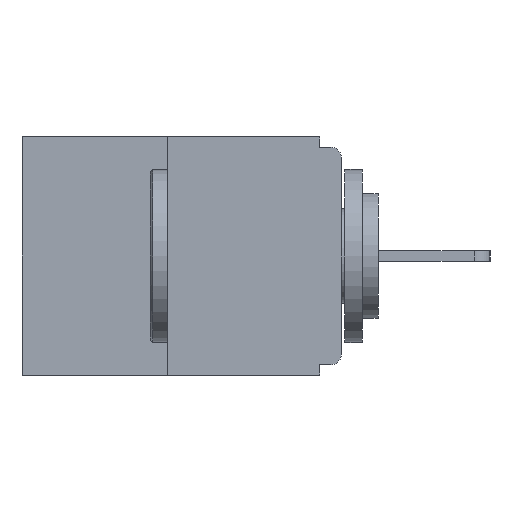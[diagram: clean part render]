
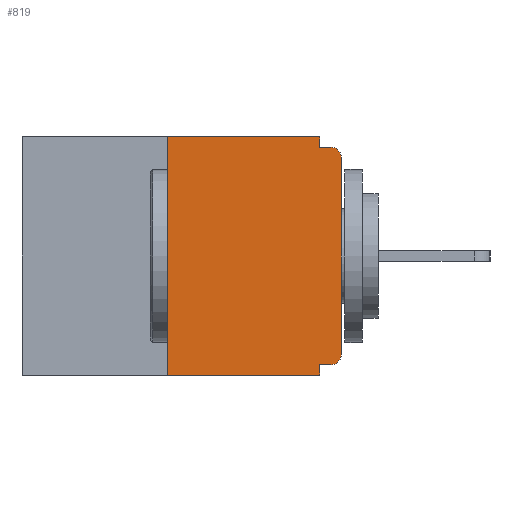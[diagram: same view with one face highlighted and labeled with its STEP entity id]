
A CAD part, left-side view. The second image highlights one B-rep face of the part: STEP entity #819.
In plain terms, the highlighted planar face has unit normal (-1, 0, 0).
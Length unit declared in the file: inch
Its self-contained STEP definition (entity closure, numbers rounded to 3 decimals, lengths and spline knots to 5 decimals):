
#14 = ORIENTED_EDGE ( 'NONE', *, *, #9934, .F. ) ;
#819 = ADVANCED_FACE ( 'NONE', ( #9322 ), #13256, .F. ) ;
#876 = ORIENTED_EDGE ( 'NONE', *, *, #11588, .F. ) ;
#1286 = LINE ( 'NONE', #10309, #9996 ) ;
#1894 = CARTESIAN_POINT ( 'NONE',  ( 0., 0., -0.015 ) ) ;
#1995 = DIRECTION ( 'NONE',  ( 0., 1., 0. ) ) ;
#2075 = EDGE_CURVE ( 'NONE', #4743, #5953, #8458, .T. ) ;
#2140 = ORIENTED_EDGE ( 'NONE', *, *, #2527, .F. ) ;
#2394 = CARTESIAN_POINT ( 'NONE',  ( 0., 0.015, -0.313 ) ) ;
#2504 = VERTEX_POINT ( 'NONE', #10908 ) ;
#2527 = EDGE_CURVE ( 'NONE', #2734, #2504, #3338, .T. ) ;
#2647 = CIRCLE ( 'NONE', #12178, 0.015 ) ;
#2734 = VERTEX_POINT ( 'NONE', #10225 ) ;
#2845 = DIRECTION ( 'NONE',  ( 0., 0., -1. ) ) ;
#3244 = ORIENTED_EDGE ( 'NONE', *, *, #14986, .T. ) ;
#3322 = EDGE_CURVE ( 'NONE', #6331, #4894, #5520, .T. ) ;
#3338 = LINE ( 'NONE', #15230, #3582 ) ;
#3570 = CARTESIAN_POINT ( 'NONE',  ( 0., 0.015, -0.015 ) ) ;
#3582 = VECTOR ( 'NONE', #4442, 39.37008 ) ;
#3686 = DIRECTION ( 'NONE',  ( 0., -1., 0. ) ) ;
#3783 = EDGE_CURVE ( 'NONE', #7012, #4894, #4788, .T. ) ;
#4094 = VECTOR ( 'NONE', #6045, 39.37008 ) ;
#4170 = CARTESIAN_POINT ( 'NONE',  ( 0., 0.031, -0.328 ) ) ;
#4374 = CARTESIAN_POINT ( 'NONE',  ( 0., 0.46, -0.343 ) ) ;
#4442 = DIRECTION ( 'NONE',  ( 0., 0., 1. ) ) ;
#4688 = ORIENTED_EDGE ( 'NONE', *, *, #3783, .F. ) ;
#4743 = VERTEX_POINT ( 'NONE', #10892 ) ;
#4788 = LINE ( 'NONE', #1894, #4094 ) ;
#4894 = VERTEX_POINT ( 'NONE', #3570 ) ;
#5467 = DIRECTION ( 'NONE',  ( 1., 0., 0. ) ) ;
#5520 = CIRCLE ( 'NONE', #15119, 0.015 ) ;
#5645 = DIRECTION ( 'NONE',  ( 0., -1., 0. ) ) ;
#5673 = VERTEX_POINT ( 'NONE', #12228 ) ;
#5953 = VERTEX_POINT ( 'NONE', #4170 ) ;
#6045 = DIRECTION ( 'NONE',  ( 0., -1., 0. ) ) ;
#6171 = VERTEX_POINT ( 'NONE', #7486 ) ;
#6331 = VERTEX_POINT ( 'NONE', #14590 ) ;
#6873 = CARTESIAN_POINT ( 'NONE',  ( 0., 0.031, 0. ) ) ;
#6968 = LINE ( 'NONE', #6873, #16480 ) ;
#7012 = VERTEX_POINT ( 'NONE', #16788 ) ;
#7073 = CARTESIAN_POINT ( 'NONE',  ( 0., 0.031, 0. ) ) ;
#7255 = VECTOR ( 'NONE', #5645, 39.37008 ) ;
#7283 = ORIENTED_EDGE ( 'NONE', *, *, #3322, .T. ) ;
#7486 = CARTESIAN_POINT ( 'NONE',  ( 0., 0.031, -0.343 ) ) ;
#7665 = AXIS2_PLACEMENT_3D ( 'NONE', #14556, #5467, #2845 ) ;
#7967 = CARTESIAN_POINT ( 'NONE',  ( 0., 0.015, -0.03 ) ) ;
#8371 = LINE ( 'NONE', #13602, #9650 ) ;
#8458 = LINE ( 'NONE', #11026, #11518 ) ;
#8956 = ORIENTED_EDGE ( 'NONE', *, *, #14340, .T. ) ;
#8972 = EDGE_CURVE ( 'NONE', #14703, #7012, #6968, .T. ) ;
#9206 = DIRECTION ( 'NONE',  ( 0., 0., -1. ) ) ;
#9322 = FACE_OUTER_BOUND ( 'NONE', #11728, .T. ) ;
#9346 = DIRECTION ( 'NONE',  ( -1., 0., 0. ) ) ;
#9544 = DIRECTION ( 'NONE',  ( 0., 0., -1. ) ) ;
#9650 = VECTOR ( 'NONE', #9747, 39.37008 ) ;
#9747 = DIRECTION ( 'NONE',  ( 0., 0., -1. ) ) ;
#9934 = EDGE_CURVE ( 'NONE', #2504, #14703, #11424, .T. ) ;
#9996 = VECTOR ( 'NONE', #15647, 39.37008 ) ;
#10201 = VECTOR ( 'NONE', #3686, 39.37008 ) ;
#10225 = CARTESIAN_POINT ( 'NONE',  ( 0., 0.25, -0.343 ) ) ;
#10309 = CARTESIAN_POINT ( 'NONE',  ( 0., 0., 0. ) ) ;
#10364 = DIRECTION ( 'NONE',  ( 0., 0., -1. ) ) ;
#10892 = CARTESIAN_POINT ( 'NONE',  ( 0., 0.015, -0.328 ) ) ;
#10908 = CARTESIAN_POINT ( 'NONE',  ( 0., 0.25, 0. ) ) ;
#11026 = CARTESIAN_POINT ( 'NONE',  ( 0., 0., -0.328 ) ) ;
#11424 = LINE ( 'NONE', #15649, #10201 ) ;
#11518 = VECTOR ( 'NONE', #1995, 39.37008 ) ;
#11588 = EDGE_CURVE ( 'NONE', #5953, #6171, #8371, .T. ) ;
#11728 = EDGE_LOOP ( 'NONE', ( #14, #2140, #8956, #876, #16757, #3244, #13403, #7283, #4688, #14796 ) ) ;
#11966 = LINE ( 'NONE', #4374, #7255 ) ;
#12178 = AXIS2_PLACEMENT_3D ( 'NONE', #2394, #13330, #9206 ) ;
#12228 = CARTESIAN_POINT ( 'NONE',  ( 0., 0., -0.313 ) ) ;
#13256 = PLANE ( 'NONE',  #7665 ) ;
#13330 = DIRECTION ( 'NONE',  ( -1., 0., 0. ) ) ;
#13403 = ORIENTED_EDGE ( 'NONE', *, *, #16213, .T. ) ;
#13602 = CARTESIAN_POINT ( 'NONE',  ( 0., 0.031, -0.343 ) ) ;
#14340 = EDGE_CURVE ( 'NONE', #2734, #6171, #11966, .T. ) ;
#14556 = CARTESIAN_POINT ( 'NONE',  ( 0., 0.46, 0. ) ) ;
#14590 = CARTESIAN_POINT ( 'NONE',  ( 0., 0., -0.03 ) ) ;
#14703 = VERTEX_POINT ( 'NONE', #7073 ) ;
#14796 = ORIENTED_EDGE ( 'NONE', *, *, #8972, .F. ) ;
#14986 = EDGE_CURVE ( 'NONE', #4743, #5673, #2647, .T. ) ;
#15119 = AXIS2_PLACEMENT_3D ( 'NONE', #7967, #9346, #10364 ) ;
#15230 = CARTESIAN_POINT ( 'NONE',  ( 0., 0.25, 0. ) ) ;
#15647 = DIRECTION ( 'NONE',  ( 0., 0., 1. ) ) ;
#15649 = CARTESIAN_POINT ( 'NONE',  ( 0., 0.46, 0. ) ) ;
#16213 = EDGE_CURVE ( 'NONE', #5673, #6331, #1286, .T. ) ;
#16480 = VECTOR ( 'NONE', #9544, 39.37008 ) ;
#16757 = ORIENTED_EDGE ( 'NONE', *, *, #2075, .F. ) ;
#16788 = CARTESIAN_POINT ( 'NONE',  ( 0., 0.031, -0.015 ) ) ;
